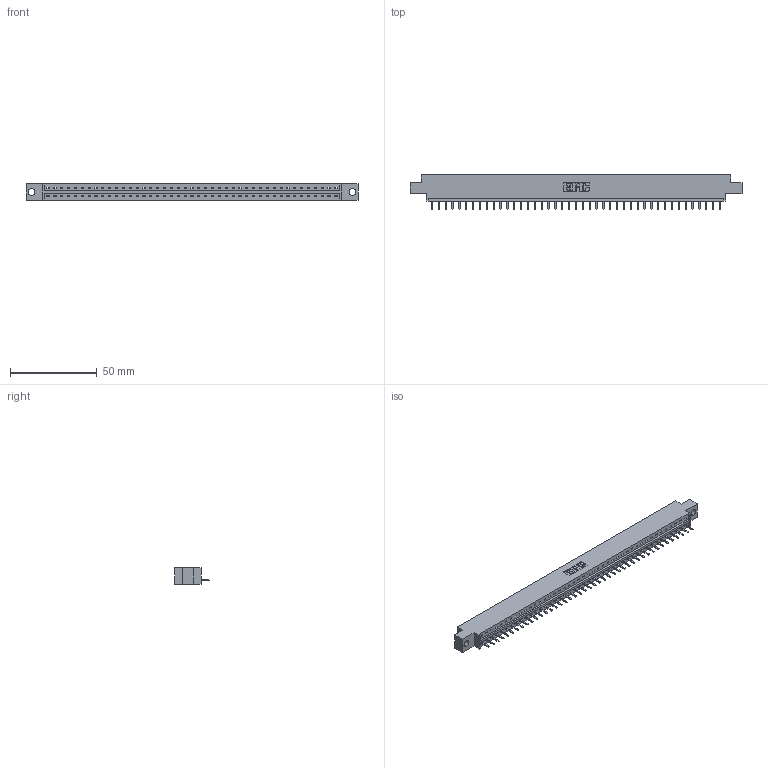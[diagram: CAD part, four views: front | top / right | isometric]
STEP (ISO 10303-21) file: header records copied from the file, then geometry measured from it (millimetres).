
FILE_DESCRIPTION (( 'STEP AP203' ), '1' );
FILE_NAME ('833-043-520-604.STEP', '2020-06-03T23:17:55', ( '' ), ( '' ), 'SwSTEP 2.0', 'SolidWorks 2020', '' );
FILE_SCHEMA (( 'CONFIG_CONTROL_DESIGN' ));
Length unit declared in the file: inch
Products named in the file (3): 345-292-001_345-293-120; 833-043-520-604; 833 Part_Offset - .156 Dia - TH
Assembly tree (44 placements, depth 2):
  833-043-520-604
    833 Part_Offset - .156 Dia - TH
    345-292-001_345-293-120  x43
Bounding box: 191.92 x 20.02 x 9.4 mm (x, y, z)
Volume: 18882.1 mm3; surface area: 19996.1 mm2
Topology: 44 solids, 44 shells, 2784 faces, 8235 edges, 5374 vertices
Faces by surface type: plane 1966, cylinder 818
Entity records: 26407 total; most frequent: CARTESIAN_POINT 4575, ORIENTED_EDGE 4542, DIRECTION 3845, EDGE_CURVE 2271, VECTOR 2139, LINE 2139, VERTEX_POINT 1510, AXIS2_PLACEMENT_3D 853
